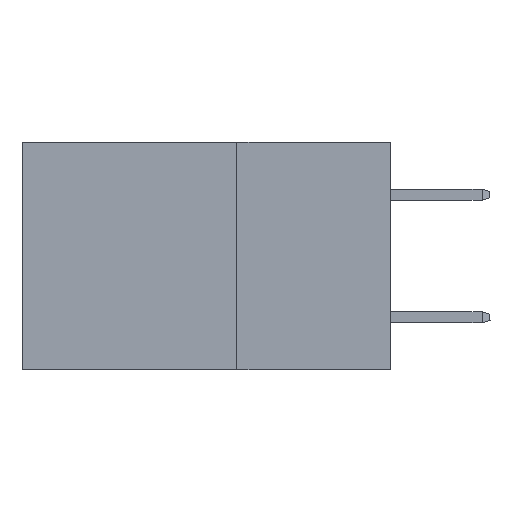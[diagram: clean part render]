
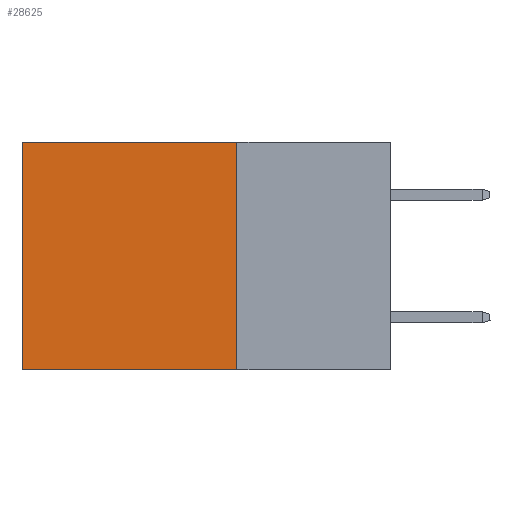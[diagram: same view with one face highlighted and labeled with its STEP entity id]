
A CAD part, left-side view. The second image highlights one B-rep face of the part: STEP entity #28625.
In plain terms, the highlighted planar face has unit normal (-1, 0, 0).
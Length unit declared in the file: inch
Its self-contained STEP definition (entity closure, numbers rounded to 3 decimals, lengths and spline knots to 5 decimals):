
#218 = VECTOR ( 'NONE', #7179, 39.37008 ) ;
#503 = VERTEX_POINT ( 'NONE', #5559 ) ;
#2227 = DIRECTION ( 'NONE',  ( 0., 0., -1. ) ) ;
#3302 = DIRECTION ( 'NONE',  ( 0., 0., -1. ) ) ;
#3443 = EDGE_CURVE ( 'NONE', #20262, #21659, #17551, .T. ) ;
#4704 = LINE ( 'NONE', #6480, #14963 ) ;
#5559 = CARTESIAN_POINT ( 'NONE',  ( 0.2875, 0.6, -0.37 ) ) ;
#6102 = VERTEX_POINT ( 'NONE', #11349 ) ;
#6229 = EDGE_CURVE ( 'NONE', #6102, #503, #15867, .T. ) ;
#6470 = CARTESIAN_POINT ( 'NONE',  ( 0.2875, 0.25, 0. ) ) ;
#6480 = CARTESIAN_POINT ( 'NONE',  ( 0.2875, 0.25, 0. ) ) ;
#7042 = EDGE_CURVE ( 'NONE', #20262, #6102, #4704, .T. ) ;
#7179 = DIRECTION ( 'NONE',  ( 0., 1., 0. ) ) ;
#7492 = CARTESIAN_POINT ( 'NONE',  ( 0.2875, 0.25, 0. ) ) ;
#7556 = LINE ( 'NONE', #16592, #23227 ) ;
#9317 = DIRECTION ( 'NONE',  ( 0., 1., 0. ) ) ;
#11349 = CARTESIAN_POINT ( 'NONE',  ( 0.2875, 0.25, -0.37 ) ) ;
#12941 = ORIENTED_EDGE ( 'NONE', *, *, #17653, .T. ) ;
#14963 = VECTOR ( 'NONE', #17562, 39.37008 ) ;
#15538 = ORIENTED_EDGE ( 'NONE', *, *, #6229, .F. ) ;
#15568 = AXIS2_PLACEMENT_3D ( 'NONE', #21097, #25777, #2227 ) ;
#15867 = LINE ( 'NONE', #24785, #25805 ) ;
#16592 = CARTESIAN_POINT ( 'NONE',  ( 0.2875, 0.6, 0. ) ) ;
#16849 = PLANE ( 'NONE',  #15568 ) ;
#17551 = LINE ( 'NONE', #6470, #218 ) ;
#17562 = DIRECTION ( 'NONE',  ( 0., 0., -1. ) ) ;
#17653 = EDGE_CURVE ( 'NONE', #21659, #503, #7556, .T. ) ;
#18587 = ORIENTED_EDGE ( 'NONE', *, *, #3443, .T. ) ;
#20137 = ORIENTED_EDGE ( 'NONE', *, *, #7042, .F. ) ;
#20262 = VERTEX_POINT ( 'NONE', #7492 ) ;
#21097 = CARTESIAN_POINT ( 'NONE',  ( 0.2875, 0.25, 0. ) ) ;
#21659 = VERTEX_POINT ( 'NONE', #25033 ) ;
#23227 = VECTOR ( 'NONE', #3302, 39.37008 ) ;
#24785 = CARTESIAN_POINT ( 'NONE',  ( 0.2875, 0.25, -0.37 ) ) ;
#25033 = CARTESIAN_POINT ( 'NONE',  ( 0.2875, 0.6, 0. ) ) ;
#25630 = FACE_OUTER_BOUND ( 'NONE', #28248, .T. ) ;
#25777 = DIRECTION ( 'NONE',  ( 1., 0., 0. ) ) ;
#25805 = VECTOR ( 'NONE', #9317, 39.37008 ) ;
#28248 = EDGE_LOOP ( 'NONE', ( #12941, #15538, #20137, #18587 ) ) ;
#28625 = ADVANCED_FACE ( 'NONE', ( #25630 ), #16849, .F. ) ;
